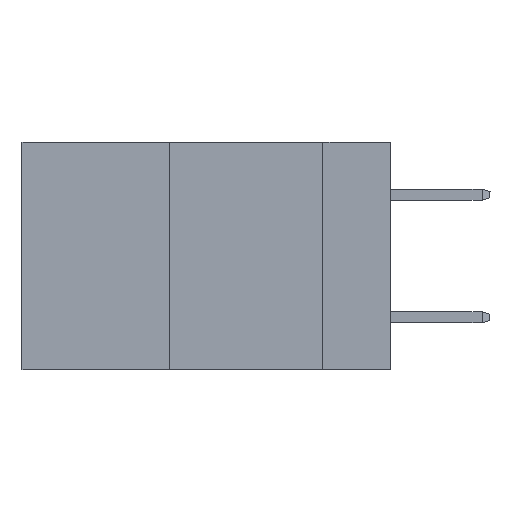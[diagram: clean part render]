
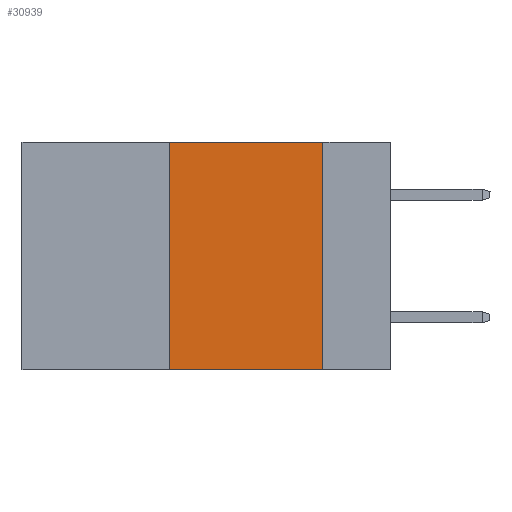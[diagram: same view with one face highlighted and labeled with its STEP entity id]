
A CAD part, left-side view. The second image highlights one B-rep face of the part: STEP entity #30939.
In plain terms, the highlighted planar face has unit normal (-1, 0, 0).
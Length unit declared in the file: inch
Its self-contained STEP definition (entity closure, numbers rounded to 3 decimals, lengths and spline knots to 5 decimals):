
#1241 = ORIENTED_EDGE ( 'NONE', *, *, #21932, .F. ) ;
#1416 = ORIENTED_EDGE ( 'NONE', *, *, #4862, .F. ) ;
#2056 = CARTESIAN_POINT ( 'NONE',  ( 0., 0.6, 0. ) ) ;
#2386 = LINE ( 'NONE', #27059, #8382 ) ;
#3059 = FACE_OUTER_BOUND ( 'NONE', #9584, .T. ) ;
#3776 = LINE ( 'NONE', #20692, #5223 ) ;
#4456 = DIRECTION ( 'NONE',  ( 1., 0., 0. ) ) ;
#4562 = ORIENTED_EDGE ( 'NONE', *, *, #22129, .F. ) ;
#4862 = EDGE_CURVE ( 'NONE', #28201, #28980, #5745, .T. ) ;
#5223 = VECTOR ( 'NONE', #27870, 39.37008 ) ;
#5745 = LINE ( 'NONE', #28471, #30973 ) ;
#8382 = VECTOR ( 'NONE', #17041, 39.37008 ) ;
#8759 = VERTEX_POINT ( 'NONE', #10083 ) ;
#9584 = EDGE_LOOP ( 'NONE', ( #1416, #4562, #1241, #26389 ) ) ;
#9862 = EDGE_CURVE ( 'NONE', #8759, #28980, #3776, .T. ) ;
#10083 = CARTESIAN_POINT ( 'NONE',  ( 0., 0.36, -0.37 ) ) ;
#12457 = CARTESIAN_POINT ( 'NONE',  ( 0., 0.11, 0. ) ) ;
#15881 = AXIS2_PLACEMENT_3D ( 'NONE', #2056, #4456, #28366 ) ;
#17041 = DIRECTION ( 'NONE',  ( 0., -1., 0. ) ) ;
#20081 = VERTEX_POINT ( 'NONE', #27137 ) ;
#20692 = CARTESIAN_POINT ( 'NONE',  ( 0., 0.6, -0.37 ) ) ;
#21080 = PLANE ( 'NONE',  #15881 ) ;
#21932 = EDGE_CURVE ( 'NONE', #8759, #20081, #22434, .T. ) ;
#22129 = EDGE_CURVE ( 'NONE', #20081, #28201, #2386, .T. ) ;
#22434 = LINE ( 'NONE', #28830, #27853 ) ;
#22583 = CARTESIAN_POINT ( 'NONE',  ( 0., 0.11, -0.37 ) ) ;
#24156 = DIRECTION ( 'NONE',  ( 0., 0., 1. ) ) ;
#26389 = ORIENTED_EDGE ( 'NONE', *, *, #9862, .T. ) ;
#27059 = CARTESIAN_POINT ( 'NONE',  ( 0., 0.6, 0. ) ) ;
#27137 = CARTESIAN_POINT ( 'NONE',  ( 0., 0.36, 0. ) ) ;
#27853 = VECTOR ( 'NONE', #24156, 39.37008 ) ;
#27870 = DIRECTION ( 'NONE',  ( 0., -1., 0. ) ) ;
#28201 = VERTEX_POINT ( 'NONE', #12457 ) ;
#28366 = DIRECTION ( 'NONE',  ( 0., 0., -1. ) ) ;
#28367 = DIRECTION ( 'NONE',  ( 0., 0., -1. ) ) ;
#28471 = CARTESIAN_POINT ( 'NONE',  ( 0., 0.11, 0. ) ) ;
#28830 = CARTESIAN_POINT ( 'NONE',  ( 0., 0.36, 0. ) ) ;
#28980 = VERTEX_POINT ( 'NONE', #22583 ) ;
#30939 = ADVANCED_FACE ( 'NONE', ( #3059 ), #21080, .F. ) ;
#30973 = VECTOR ( 'NONE', #28367, 39.37008 ) ;
